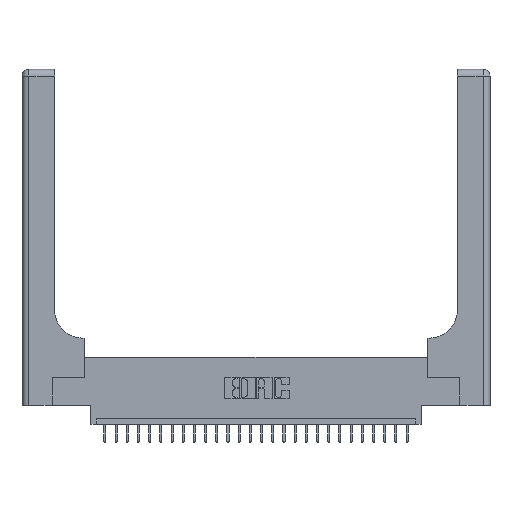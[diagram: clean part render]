
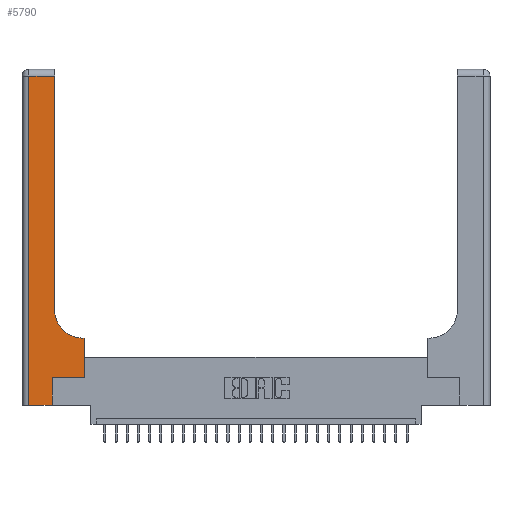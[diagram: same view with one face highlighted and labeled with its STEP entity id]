
A CAD part, top view. The second image highlights one B-rep face of the part: STEP entity #5790.
In plain terms, the highlighted planar face has unit normal (0, 0, 1).
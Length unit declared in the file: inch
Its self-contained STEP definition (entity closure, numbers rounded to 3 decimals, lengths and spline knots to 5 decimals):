
#110 = VERTEX_POINT ( 'NONE', #6693 ) ;
#386 = CARTESIAN_POINT ( 'NONE',  ( 0.06, 0., 0.37 ) ) ;
#393 = LINE ( 'NONE', #18796, #15886 ) ;
#1032 = LINE ( 'NONE', #4361, #17878 ) ;
#1682 = EDGE_LOOP ( 'NONE', ( #5941, #15848, #15570, #3383, #18111, #14742, #14892, #20681, #21733 ) ) ;
#1722 = LINE ( 'NONE', #27208, #9999 ) ;
#2038 = LINE ( 'NONE', #8699, #15138 ) ;
#2173 = CARTESIAN_POINT ( 'NONE',  ( 0.06, 3., 0.37 ) ) ;
#2264 = DIRECTION ( 'NONE',  ( -1., 0., 0. ) ) ;
#2343 = DIRECTION ( 'NONE',  ( 0., 1., 0. ) ) ;
#2378 = CARTESIAN_POINT ( 'NONE',  ( 0.5415, 0.6, 0.37 ) ) ;
#2821 = LINE ( 'NONE', #22083, #22719 ) ;
#3383 = ORIENTED_EDGE ( 'NONE', *, *, #12558, .T. ) ;
#3633 = CARTESIAN_POINT ( 'NONE',  ( 0., 3., 0.37 ) ) ;
#4361 = CARTESIAN_POINT ( 'NONE',  ( 0.2915, 3., 0.37 ) ) ;
#4738 = DIRECTION ( 'NONE',  ( 0., -1., 0. ) ) ;
#4758 = EDGE_CURVE ( 'NONE', #24810, #27183, #26509, .T. ) ;
#5473 = CIRCLE ( 'NONE', #22451, 0.25 ) ;
#5603 = LINE ( 'NONE', #5872, #6296 ) ;
#5790 = ADVANCED_FACE ( 'NONE', ( #15875 ), #25490, .F. ) ;
#5872 = CARTESIAN_POINT ( 'NONE',  ( 0.269, 0., 0.37 ) ) ;
#5941 = ORIENTED_EDGE ( 'NONE', *, *, #12679, .T. ) ;
#6296 = VECTOR ( 'NONE', #23515, 39.37008 ) ;
#6693 = CARTESIAN_POINT ( 'NONE',  ( 0.2915, 2.94, 0.37 ) ) ;
#8200 = DIRECTION ( 'NONE',  ( 0., 0., -1. ) ) ;
#8699 = CARTESIAN_POINT ( 'NONE',  ( 0., 2.94, 0.37 ) ) ;
#9765 = CARTESIAN_POINT ( 'NONE',  ( 0.5585, 0.6, 0.37 ) ) ;
#9999 = VECTOR ( 'NONE', #27009, 39.37008 ) ;
#10185 = VERTEX_POINT ( 'NONE', #23157 ) ;
#11124 = EDGE_CURVE ( 'NONE', #16556, #20195, #27527, .T. ) ;
#12306 = DIRECTION ( 'NONE',  ( 0., 0., -1. ) ) ;
#12558 = EDGE_CURVE ( 'NONE', #27183, #21424, #1722, .T. ) ;
#12572 = DIRECTION ( 'NONE',  ( 0., 1., 0. ) ) ;
#12679 = EDGE_CURVE ( 'NONE', #10185, #110, #1032, .T. ) ;
#12684 = EDGE_CURVE ( 'NONE', #110, #24810, #2038, .T. ) ;
#14009 = CARTESIAN_POINT ( 'NONE',  ( 0.269, 0.25, 0.37 ) ) ;
#14742 = ORIENTED_EDGE ( 'NONE', *, *, #14961, .T. ) ;
#14892 = ORIENTED_EDGE ( 'NONE', *, *, #25651, .T. ) ;
#14957 = DIRECTION ( 'NONE',  ( 1., 0., 0. ) ) ;
#14961 = EDGE_CURVE ( 'NONE', #16393, #24405, #2821, .T. ) ;
#15138 = VECTOR ( 'NONE', #2264, 39.37008 ) ;
#15443 = CARTESIAN_POINT ( 'NONE',  ( 0.5415, 0.85, 0.37 ) ) ;
#15535 = DIRECTION ( 'NONE',  ( -1., 0., 0. ) ) ;
#15570 = ORIENTED_EDGE ( 'NONE', *, *, #4758, .T. ) ;
#15848 = ORIENTED_EDGE ( 'NONE', *, *, #12684, .T. ) ;
#15875 = FACE_OUTER_BOUND ( 'NONE', #1682, .T. ) ;
#15886 = VECTOR ( 'NONE', #12572, 39.37008 ) ;
#16393 = VERTEX_POINT ( 'NONE', #14009 ) ;
#16556 = VERTEX_POINT ( 'NONE', #9765 ) ;
#17188 = EDGE_CURVE ( 'NONE', #20195, #10185, #5473, .T. ) ;
#17700 = DIRECTION ( 'NONE',  ( 1., 0., 0. ) ) ;
#17878 = VECTOR ( 'NONE', #2343, 39.37008 ) ;
#18111 = ORIENTED_EDGE ( 'NONE', *, *, #24348, .T. ) ;
#18796 = CARTESIAN_POINT ( 'NONE',  ( 0.5585, 0.25, 0.37 ) ) ;
#19304 = VECTOR ( 'NONE', #4738, 39.37008 ) ;
#19853 = CARTESIAN_POINT ( 'NONE',  ( 0.06, 2.94, 0.37 ) ) ;
#20075 = AXIS2_PLACEMENT_3D ( 'NONE', #3633, #12306, #23382 ) ;
#20195 = VERTEX_POINT ( 'NONE', #2378 ) ;
#20206 = CARTESIAN_POINT ( 'NONE',  ( 0.269, 0., 0.37 ) ) ;
#20681 = ORIENTED_EDGE ( 'NONE', *, *, #11124, .T. ) ;
#21058 = VECTOR ( 'NONE', #15535, 39.37008 ) ;
#21424 = VERTEX_POINT ( 'NONE', #20206 ) ;
#21733 = ORIENTED_EDGE ( 'NONE', *, *, #17188, .T. ) ;
#22083 = CARTESIAN_POINT ( 'NONE',  ( 0.269, 0.25, 0.37 ) ) ;
#22451 = AXIS2_PLACEMENT_3D ( 'NONE', #15443, #8200, #14957 ) ;
#22719 = VECTOR ( 'NONE', #17700, 39.37008 ) ;
#23157 = CARTESIAN_POINT ( 'NONE',  ( 0.2915, 0.85, 0.37 ) ) ;
#23382 = DIRECTION ( 'NONE',  ( -1., 0., 0. ) ) ;
#23515 = DIRECTION ( 'NONE',  ( 0., 1., 0. ) ) ;
#24348 = EDGE_CURVE ( 'NONE', #21424, #16393, #5603, .T. ) ;
#24405 = VERTEX_POINT ( 'NONE', #27131 ) ;
#24810 = VERTEX_POINT ( 'NONE', #19853 ) ;
#25490 = PLANE ( 'NONE',  #20075 ) ;
#25651 = EDGE_CURVE ( 'NONE', #24405, #16556, #393, .T. ) ;
#25916 = CARTESIAN_POINT ( 'NONE',  ( 0.2915, 0.6, 0.37 ) ) ;
#26509 = LINE ( 'NONE', #2173, #19304 ) ;
#27009 = DIRECTION ( 'NONE',  ( 1., 0., 0. ) ) ;
#27131 = CARTESIAN_POINT ( 'NONE',  ( 0.5585, 0.25, 0.37 ) ) ;
#27183 = VERTEX_POINT ( 'NONE', #386 ) ;
#27208 = CARTESIAN_POINT ( 'NONE',  ( 0., 0., 0.37 ) ) ;
#27527 = LINE ( 'NONE', #25916, #21058 ) ;
